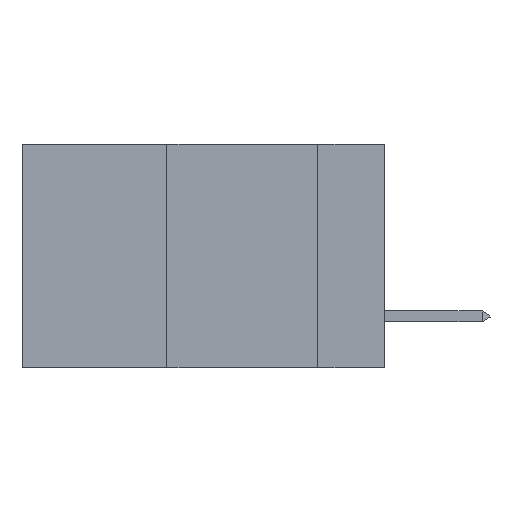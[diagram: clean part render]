
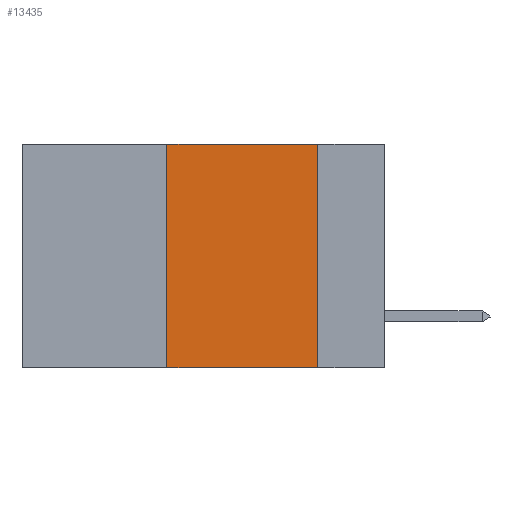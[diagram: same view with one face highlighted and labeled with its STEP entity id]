
A CAD part, left-side view. The second image highlights one B-rep face of the part: STEP entity #13435.
In plain terms, the highlighted planar face has unit normal (-1, 0, 0).
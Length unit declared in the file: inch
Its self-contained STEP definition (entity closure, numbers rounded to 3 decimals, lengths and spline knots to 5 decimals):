
#348 = VECTOR ( 'NONE', #26451, 39.37008 ) ;
#1635 = EDGE_CURVE ( 'NONE', #26169, #29276, #19256, .T. ) ;
#1883 = LINE ( 'NONE', #25289, #10648 ) ;
#2643 = DIRECTION ( 'NONE',  ( 0., 0., -1. ) ) ;
#2771 = CARTESIAN_POINT ( 'NONE',  ( 0., 0.6, 0. ) ) ;
#2873 = AXIS2_PLACEMENT_3D ( 'NONE', #2771, #8341, #2643 ) ;
#3018 = CARTESIAN_POINT ( 'NONE',  ( 0., 0.11, 0. ) ) ;
#6127 = EDGE_CURVE ( 'NONE', #27049, #22236, #1883, .T. ) ;
#6352 = CARTESIAN_POINT ( 'NONE',  ( 0., 0.36, 0. ) ) ;
#6718 = FACE_OUTER_BOUND ( 'NONE', #8881, .T. ) ;
#8341 = DIRECTION ( 'NONE',  ( 1., 0., 0. ) ) ;
#8881 = EDGE_LOOP ( 'NONE', ( #34255, #19898, #12750, #25468 ) ) ;
#10648 = VECTOR ( 'NONE', #22182, 39.37008 ) ;
#10796 = DIRECTION ( 'NONE',  ( 0., -1., 0. ) ) ;
#11206 = LINE ( 'NONE', #25549, #33636 ) ;
#12553 = EDGE_CURVE ( 'NONE', #29276, #27049, #13281, .T. ) ;
#12750 = ORIENTED_EDGE ( 'NONE', *, *, #1635, .F. ) ;
#13281 = LINE ( 'NONE', #34948, #348 ) ;
#13435 = ADVANCED_FACE ( 'NONE', ( #6718 ), #34879, .F. ) ;
#13498 = CARTESIAN_POINT ( 'NONE',  ( 0., 0.36, 0. ) ) ;
#15958 = EDGE_CURVE ( 'NONE', #26169, #22236, #11206, .T. ) ;
#17238 = CARTESIAN_POINT ( 'NONE',  ( 0., 0.36, -0.37 ) ) ;
#19256 = LINE ( 'NONE', #6352, #34895 ) ;
#19898 = ORIENTED_EDGE ( 'NONE', *, *, #12553, .F. ) ;
#20575 = DIRECTION ( 'NONE',  ( 0., 0., 1. ) ) ;
#22182 = DIRECTION ( 'NONE',  ( 0., 0., -1. ) ) ;
#22236 = VERTEX_POINT ( 'NONE', #27376 ) ;
#25289 = CARTESIAN_POINT ( 'NONE',  ( 0., 0.11, 0. ) ) ;
#25468 = ORIENTED_EDGE ( 'NONE', *, *, #15958, .T. ) ;
#25549 = CARTESIAN_POINT ( 'NONE',  ( 0., 0.6, -0.37 ) ) ;
#26169 = VERTEX_POINT ( 'NONE', #17238 ) ;
#26451 = DIRECTION ( 'NONE',  ( 0., -1., 0. ) ) ;
#27049 = VERTEX_POINT ( 'NONE', #3018 ) ;
#27376 = CARTESIAN_POINT ( 'NONE',  ( 0., 0.11, -0.37 ) ) ;
#29276 = VERTEX_POINT ( 'NONE', #13498 ) ;
#33636 = VECTOR ( 'NONE', #10796, 39.37008 ) ;
#34255 = ORIENTED_EDGE ( 'NONE', *, *, #6127, .F. ) ;
#34879 = PLANE ( 'NONE',  #2873 ) ;
#34895 = VECTOR ( 'NONE', #20575, 39.37008 ) ;
#34948 = CARTESIAN_POINT ( 'NONE',  ( 0., 0.6, 0. ) ) ;
